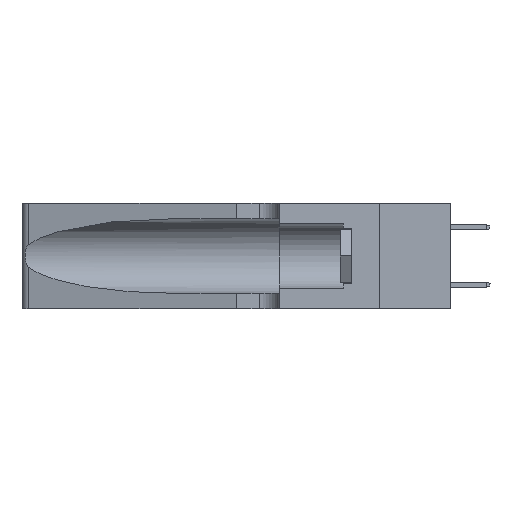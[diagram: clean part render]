
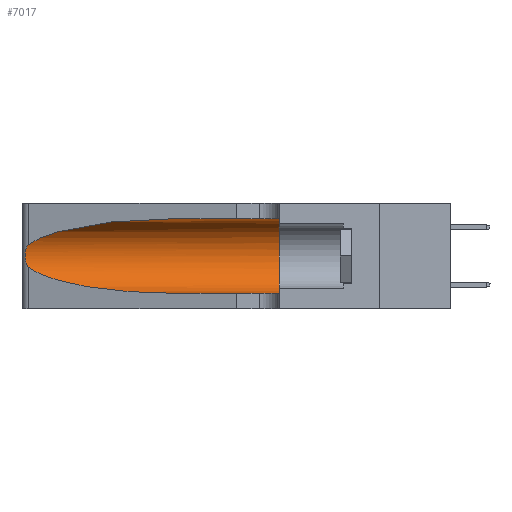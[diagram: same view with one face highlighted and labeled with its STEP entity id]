
A CAD part, left-side view. The second image highlights one B-rep face of the part: STEP entity #7017.
In plain terms, the highlighted cylindrical face has radius 3.308 mm (diameter 6.617 mm), a partial arc.
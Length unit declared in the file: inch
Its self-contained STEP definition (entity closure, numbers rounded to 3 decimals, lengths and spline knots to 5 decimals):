
#569 = EDGE_LOOP ( 'NONE', ( #19891, #2827, #1058, #6078, #12383, #28742 ) ) ;
#1058 = ORIENTED_EDGE ( 'NONE', *, *, #37201, .T. ) ;
#1248 = CIRCLE ( 'NONE', #33769, 0.13025 ) ;
#1370 = DIRECTION ( 'NONE',  ( 0., 0., -1. ) ) ;
#1591 = VERTEX_POINT ( 'NONE', #2017 ) ;
#2017 = CARTESIAN_POINT ( 'NONE',  ( 0.1305, 0.72297, 0.31525 ) ) ;
#2483 = DIRECTION ( 'NONE',  ( 0., -1., 0. ) ) ;
#2827 = ORIENTED_EDGE ( 'NONE', *, *, #12809, .T. ) ;
#3043 = CARTESIAN_POINT ( 'NONE',  ( 0.1305, 0.72297, 0.05475 ) ) ;
#6078 = ORIENTED_EDGE ( 'NONE', *, *, #10897, .T. ) ;
#6516 = CARTESIAN_POINT ( 'NONE',  ( 0.25487, 1.22718, 0.22369 ) ) ;
#6653 = AXIS2_PLACEMENT_3D ( 'NONE', #26539, #10718, #1370 ) ;
#6755 = CARTESIAN_POINT ( 'NONE',  ( 0.26075, 1.23896, 0.19203 ) ) ;
#7017 = ADVANCED_FACE ( 'NONE', ( #30456 ), #13829, .F. ) ;
#7593 =( BOUNDED_CURVE ( )  B_SPLINE_CURVE ( 3, ( #37300, #27932, #31250, #6516 ),
 .UNSPECIFIED., .F., .F. ) 
 B_SPLINE_CURVE_WITH_KNOTS ( ( 4, 4 ),
 ( 1.5708, 2.84003 ),
 .UNSPECIFIED. ) 
 CURVE ( )  GEOMETRIC_REPRESENTATION_ITEM ( )  RATIONAL_B_SPLINE_CURVE ( ( 1., 0.87, 0.87, 1. ) ) 
 REPRESENTATION_ITEM ( '' )  );
#7986 = VECTOR ( 'NONE', #2483, 39.37008 ) ;
#8174 = VECTOR ( 'NONE', #30205, 39.37008 ) ;
#8901 = CARTESIAN_POINT ( 'NONE',  ( 0.1305, 0.72297, 0.05475 ) ) ;
#9272 = EDGE_CURVE ( 'NONE', #9848, #9897, #1248, .T. ) ;
#9696 = EDGE_CURVE ( 'NONE', #1591, #28482, #7593, .T. ) ;
#9848 = VERTEX_POINT ( 'NONE', #13363 ) ;
#9863 = CARTESIAN_POINT ( 'NONE',  ( 0.25854, 1.2359, 0.20912 ) ) ;
#9897 = VERTEX_POINT ( 'NONE', #32714 ) ;
#10574 = CARTESIAN_POINT ( 'NONE',  ( 0.1305, 0.35, 0.185 ) ) ;
#10718 = DIRECTION ( 'NONE',  ( 0., -1., 0. ) ) ;
#10897 = EDGE_CURVE ( 'NONE', #11423, #9897, #17497, .T. ) ;
#11423 = VERTEX_POINT ( 'NONE', #8901 ) ;
#11674 = CARTESIAN_POINT ( 'NONE',  ( 0.1305, 1.61858, 0.05475 ) ) ;
#12383 = ORIENTED_EDGE ( 'NONE', *, *, #9272, .F. ) ;
#12809 = EDGE_CURVE ( 'NONE', #28482, #17761, #29423, .T. ) ;
#12985 = CARTESIAN_POINT ( 'NONE',  ( 0.25639, 1.23184, 0.21858 ) ) ;
#13363 = CARTESIAN_POINT ( 'NONE',  ( 0.1305, 0.35, 0.31525 ) ) ;
#13390 = CARTESIAN_POINT ( 'NONE',  ( 0.25789, 1.23486, 0.15765 ) ) ;
#13829 = CYLINDRICAL_SURFACE ( 'NONE', #6653, 0.13025 ) ;
#13995 = CARTESIAN_POINT ( 'NONE',  ( 0.25487, 1.22718, 0.14631 ) ) ;
#15847 = EDGE_CURVE ( 'NONE', #1591, #9848, #28270, .T. ) ;
#16496 = CARTESIAN_POINT ( 'NONE',  ( 0.25639, 1.23186, 0.15144 ) ) ;
#17497 = LINE ( 'NONE', #11674, #8174 ) ;
#17761 = VERTEX_POINT ( 'NONE', #29136 ) ;
#19419 = CARTESIAN_POINT ( 'NONE',  ( 0.26075, 1.23896, 0.178 ) ) ;
#19891 = ORIENTED_EDGE ( 'NONE', *, *, #9696, .T. ) ;
#20144 = DIRECTION ( 'NONE',  ( 0., 1., 0. ) ) ;
#21148 = CARTESIAN_POINT ( 'NONE',  ( 0.2373, 1.15595, 0.08982 ) ) ;
#21342 = CARTESIAN_POINT ( 'NONE',  ( 0.18966, 0.96281, 0.05475 ) ) ;
#22132 = CARTESIAN_POINT ( 'NONE',  ( 0.25787, 1.23484, 0.2124 ) ) ;
#23569 = CARTESIAN_POINT ( 'NONE',  ( 0.25555, 1.22993, 0.14849 ) ) ;
#25141 = CARTESIAN_POINT ( 'NONE',  ( 0.1305, 1.61858, 0.31525 ) ) ;
#26539 = CARTESIAN_POINT ( 'NONE',  ( 0.1305, 1.61858, 0.185 ) ) ;
#27932 = CARTESIAN_POINT ( 'NONE',  ( 0.18966, 0.96281, 0.31525 ) ) ;
#28270 = LINE ( 'NONE', #25141, #7986 ) ;
#28482 = VERTEX_POINT ( 'NONE', #36118 ) ;
#28742 = ORIENTED_EDGE ( 'NONE', *, *, #15847, .F. ) ;
#28801 = CARTESIAN_POINT ( 'NONE',  ( 0.25487, 1.22718, 0.22369 ) ) ;
#29004 = CARTESIAN_POINT ( 'NONE',  ( 0.26017, 1.23833, 0.17102 ) ) ;
#29136 = CARTESIAN_POINT ( 'NONE',  ( 0.25487, 1.22718, 0.14631 ) ) ;
#29423 = B_SPLINE_CURVE_WITH_KNOTS ( 'NONE', 3,
 ( #28801, #41056, #12985, #22132, #9863, #35261, #6755, #19419, #29004, #38599, #13390, #16496, #23569, #13995 ),
 .UNSPECIFIED., .F., .F.,
 ( 4, 2, 2, 2, 2, 2, 4 ),
 ( 0., 0.00027, 0.00053, 0.00107, 0.0016, 0.00187, 0.00214 ),
 .UNSPECIFIED. ) ;
#30205 = DIRECTION ( 'NONE',  ( 0., -1., 0. ) ) ;
#30456 = FACE_OUTER_BOUND ( 'NONE', #569, .T. ) ;
#31250 = CARTESIAN_POINT ( 'NONE',  ( 0.2373, 1.15595, 0.28018 ) ) ;
#32714 = CARTESIAN_POINT ( 'NONE',  ( 0.1305, 0.35, 0.05475 ) ) ;
#32845 = DIRECTION ( 'NONE',  ( 0., 0., 1. ) ) ;
#33121 =( BOUNDED_CURVE ( )  B_SPLINE_CURVE ( 3, ( #34251, #21148, #21342, #3043 ),
 .UNSPECIFIED., .F., .F. ) 
 B_SPLINE_CURVE_WITH_KNOTS ( ( 4, 4 ),
 ( 3.44316, 4.71239 ),
 .UNSPECIFIED. ) 
 CURVE ( )  GEOMETRIC_REPRESENTATION_ITEM ( )  RATIONAL_B_SPLINE_CURVE ( ( 1., 0.87, 0.87, 1. ) ) 
 REPRESENTATION_ITEM ( '' )  );
#33769 = AXIS2_PLACEMENT_3D ( 'NONE', #10574, #20144, #32845 ) ;
#34251 = CARTESIAN_POINT ( 'NONE',  ( 0.25487, 1.22718, 0.14631 ) ) ;
#35261 = CARTESIAN_POINT ( 'NONE',  ( 0.26018, 1.23835, 0.19895 ) ) ;
#36118 = CARTESIAN_POINT ( 'NONE',  ( 0.25487, 1.22718, 0.22369 ) ) ;
#37201 = EDGE_CURVE ( 'NONE', #17761, #11423, #33121, .T. ) ;
#37300 = CARTESIAN_POINT ( 'NONE',  ( 0.1305, 0.72297, 0.31525 ) ) ;
#38599 = CARTESIAN_POINT ( 'NONE',  ( 0.25856, 1.23593, 0.16098 ) ) ;
#41056 = CARTESIAN_POINT ( 'NONE',  ( 0.25555, 1.22994, 0.2215 ) ) ;
